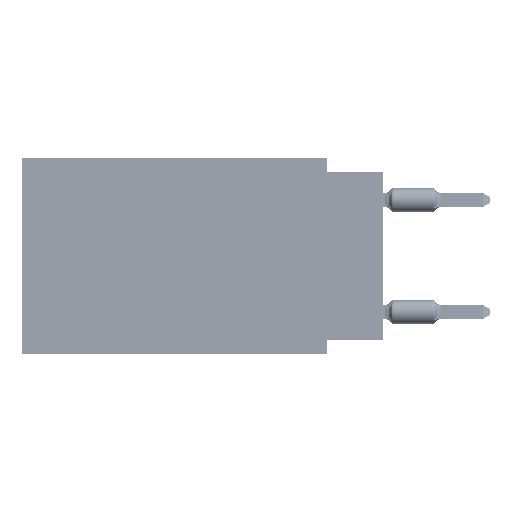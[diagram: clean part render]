
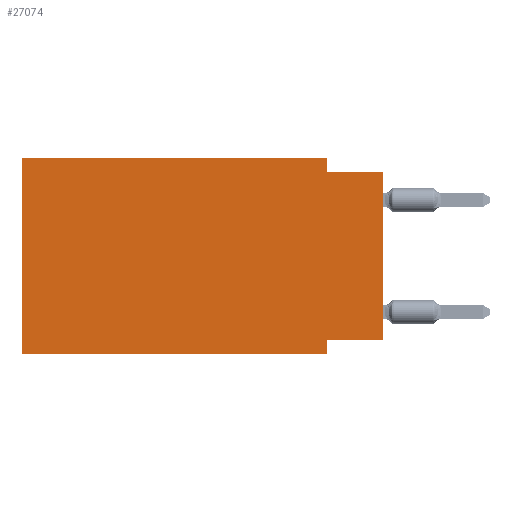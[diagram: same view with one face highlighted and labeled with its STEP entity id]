
A CAD part, left-side view. The second image highlights one B-rep face of the part: STEP entity #27074.
In plain terms, the highlighted planar face has unit normal (-1, 0, 0).
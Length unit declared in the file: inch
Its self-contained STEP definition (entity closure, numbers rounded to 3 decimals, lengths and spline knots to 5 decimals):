
#427 = CARTESIAN_POINT ( 'NONE',  ( 0., 0.645, 0. ) ) ;
#1681 = ORIENTED_EDGE ( 'NONE', *, *, #52896, .T. ) ;
#2325 = VECTOR ( 'NONE', #37602, 39.37008 ) ;
#2404 = VERTEX_POINT ( 'NONE', #53312 ) ;
#2805 = EDGE_CURVE ( 'NONE', #2404, #66551, #65262, .T. ) ;
#3187 = LINE ( 'NONE', #56620, #5351 ) ;
#3615 = DIRECTION ( 'NONE',  ( 0., 1., 0. ) ) ;
#4296 = LINE ( 'NONE', #53754, #18398 ) ;
#4335 = LINE ( 'NONE', #43386, #20136 ) ;
#4474 = CARTESIAN_POINT ( 'NONE',  ( 0., 0.1, -0.325 ) ) ;
#5351 = VECTOR ( 'NONE', #63018, 39.37008 ) ;
#5747 = EDGE_CURVE ( 'NONE', #66551, #56305, #63966, .T. ) ;
#5800 = CARTESIAN_POINT ( 'NONE',  ( 0., 0.645, 0. ) ) ;
#5855 = LINE ( 'NONE', #11935, #38404 ) ;
#11935 = CARTESIAN_POINT ( 'NONE',  ( 0., 0.645, -0.35 ) ) ;
#13881 = ORIENTED_EDGE ( 'NONE', *, *, #35360, .F. ) ;
#14370 = VERTEX_POINT ( 'NONE', #21167 ) ;
#15746 = LINE ( 'NONE', #65152, #2325 ) ;
#18398 = VECTOR ( 'NONE', #64811, 39.37008 ) ;
#20136 = VECTOR ( 'NONE', #69891, 39.37008 ) ;
#21167 = CARTESIAN_POINT ( 'NONE',  ( 0., 0.1, -0.025 ) ) ;
#21173 = CARTESIAN_POINT ( 'NONE',  ( 0., 0., -0.025 ) ) ;
#21599 = VERTEX_POINT ( 'NONE', #62037 ) ;
#24065 = CARTESIAN_POINT ( 'NONE',  ( 0., 0., -0.325 ) ) ;
#24121 = EDGE_LOOP ( 'NONE', ( #43223, #60672, #32026, #34449, #29137, #1681, #13881, #55874 ) ) ;
#25176 = VECTOR ( 'NONE', #3615, 39.37008 ) ;
#27074 = ADVANCED_FACE ( 'NONE', ( #33028 ), #48468, .F. ) ;
#29137 = ORIENTED_EDGE ( 'NONE', *, *, #2805, .F. ) ;
#29185 = VECTOR ( 'NONE', #54205, 39.37008 ) ;
#30559 = VERTEX_POINT ( 'NONE', #60176 ) ;
#30916 = CARTESIAN_POINT ( 'NONE',  ( 0., 0.645, 0. ) ) ;
#32026 = ORIENTED_EDGE ( 'NONE', *, *, #67094, .F. ) ;
#33028 = FACE_OUTER_BOUND ( 'NONE', #24121, .T. ) ;
#33450 = DIRECTION ( 'NONE',  ( 0., -1., 0. ) ) ;
#34449 = ORIENTED_EDGE ( 'NONE', *, *, #5747, .F. ) ;
#35360 = EDGE_CURVE ( 'NONE', #68475, #30559, #15746, .T. ) ;
#37602 = DIRECTION ( 'NONE',  ( 0., 0., -1. ) ) ;
#38404 = VECTOR ( 'NONE', #33450, 39.37008 ) ;
#38764 = DIRECTION ( 'NONE',  ( 0., 0., -1. ) ) ;
#39138 = LINE ( 'NONE', #24065, #25176 ) ;
#41798 = DIRECTION ( 'NONE',  ( 0., -1., 0. ) ) ;
#42446 = VECTOR ( 'NONE', #41798, 39.37008 ) ;
#43223 = ORIENTED_EDGE ( 'NONE', *, *, #54028, .T. ) ;
#43386 = CARTESIAN_POINT ( 'NONE',  ( 0., 0., -0.025 ) ) ;
#48468 = PLANE ( 'NONE',  #52957 ) ;
#49404 = VERTEX_POINT ( 'NONE', #21173 ) ;
#51544 = EDGE_CURVE ( 'NONE', #14370, #49404, #4335, .T. ) ;
#52896 = EDGE_CURVE ( 'NONE', #2404, #30559, #5855, .T. ) ;
#52957 = AXIS2_PLACEMENT_3D ( 'NONE', #5800, #70290, #38764 ) ;
#53312 = CARTESIAN_POINT ( 'NONE',  ( 0., 0.645, -0.35 ) ) ;
#53612 = CARTESIAN_POINT ( 'NONE',  ( 0., 0.645, 0. ) ) ;
#53754 = CARTESIAN_POINT ( 'NONE',  ( 0., 0.1, 0. ) ) ;
#54028 = EDGE_CURVE ( 'NONE', #21599, #49404, #3187, .T. ) ;
#54205 = DIRECTION ( 'NONE',  ( 0., 0., 1. ) ) ;
#55874 = ORIENTED_EDGE ( 'NONE', *, *, #62000, .F. ) ;
#56305 = VERTEX_POINT ( 'NONE', #57324 ) ;
#56620 = CARTESIAN_POINT ( 'NONE',  ( 0., 0., 0. ) ) ;
#57324 = CARTESIAN_POINT ( 'NONE',  ( 0., 0.1, 0. ) ) ;
#60176 = CARTESIAN_POINT ( 'NONE',  ( 0., 0.1, -0.35 ) ) ;
#60672 = ORIENTED_EDGE ( 'NONE', *, *, #51544, .F. ) ;
#62000 = EDGE_CURVE ( 'NONE', #21599, #68475, #39138, .T. ) ;
#62037 = CARTESIAN_POINT ( 'NONE',  ( 0., 0., -0.325 ) ) ;
#63018 = DIRECTION ( 'NONE',  ( 0., 0., 1. ) ) ;
#63966 = LINE ( 'NONE', #53612, #42446 ) ;
#64811 = DIRECTION ( 'NONE',  ( 0., 0., -1. ) ) ;
#65152 = CARTESIAN_POINT ( 'NONE',  ( 0., 0.1, -0.35 ) ) ;
#65262 = LINE ( 'NONE', #427, #29185 ) ;
#66551 = VERTEX_POINT ( 'NONE', #30916 ) ;
#67094 = EDGE_CURVE ( 'NONE', #56305, #14370, #4296, .T. ) ;
#68475 = VERTEX_POINT ( 'NONE', #4474 ) ;
#69891 = DIRECTION ( 'NONE',  ( 0., -1., 0. ) ) ;
#70290 = DIRECTION ( 'NONE',  ( 1., 0., 0. ) ) ;
